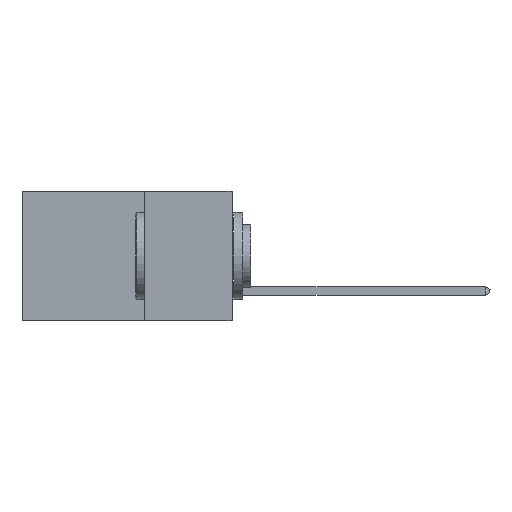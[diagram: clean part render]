
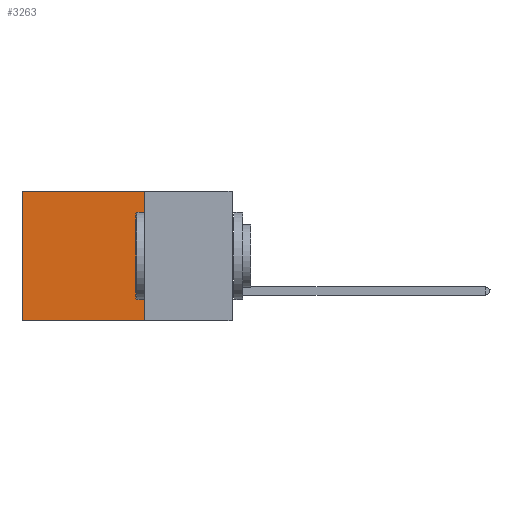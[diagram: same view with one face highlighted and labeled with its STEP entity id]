
A CAD part, left-side view. The second image highlights one B-rep face of the part: STEP entity #3263.
In plain terms, the highlighted planar face has unit normal (-1, 0, 0).
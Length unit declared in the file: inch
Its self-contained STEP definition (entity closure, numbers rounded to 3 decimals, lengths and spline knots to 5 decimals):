
#88 = VERTEX_POINT ( 'NONE', #1532 ) ;
#314 = EDGE_CURVE ( 'NONE', #6139, #6367, #6616, .T. ) ;
#353 = AXIS2_PLACEMENT_3D ( 'NONE', #1409, #7370, #13985 ) ;
#774 = EDGE_LOOP ( 'NONE', ( #6247, #1209, #3418, #14110 ) ) ;
#1006 = CARTESIAN_POINT ( 'NONE',  ( 0.2875, 0.25, 0. ) ) ;
#1209 = ORIENTED_EDGE ( 'NONE', *, *, #1333, .F. ) ;
#1333 = EDGE_CURVE ( 'NONE', #7862, #88, #13967, .T. ) ;
#1409 = CARTESIAN_POINT ( 'NONE',  ( 0.2875, 0.25, 0. ) ) ;
#1532 = CARTESIAN_POINT ( 'NONE',  ( 0.2875, 0.6, -0.37 ) ) ;
#1663 = DIRECTION ( 'NONE',  ( 0., 0., -1. ) ) ;
#1742 = VECTOR ( 'NONE', #6605, 39.37008 ) ;
#2166 = EDGE_CURVE ( 'NONE', #6139, #7862, #2516, .T. ) ;
#2516 = LINE ( 'NONE', #9166, #11994 ) ;
#2729 = CARTESIAN_POINT ( 'NONE',  ( 0.2875, 0.25, 0. ) ) ;
#2847 = CARTESIAN_POINT ( 'NONE',  ( 0.2875, 0.25, -0.37 ) ) ;
#3263 = ADVANCED_FACE ( 'NONE', ( #13203 ), #6681, .F. ) ;
#3418 = ORIENTED_EDGE ( 'NONE', *, *, #2166, .F. ) ;
#4540 = EDGE_CURVE ( 'NONE', #6367, #88, #7748, .T. ) ;
#4544 = VECTOR ( 'NONE', #9429, 39.37008 ) ;
#6139 = VERTEX_POINT ( 'NONE', #1006 ) ;
#6228 = DIRECTION ( 'NONE',  ( 0., 1., 0. ) ) ;
#6247 = ORIENTED_EDGE ( 'NONE', *, *, #4540, .T. ) ;
#6367 = VERTEX_POINT ( 'NONE', #10003 ) ;
#6605 = DIRECTION ( 'NONE',  ( 0., 0., -1. ) ) ;
#6616 = LINE ( 'NONE', #2729, #10501 ) ;
#6681 = PLANE ( 'NONE',  #353 ) ;
#7370 = DIRECTION ( 'NONE',  ( 1., 0., 0. ) ) ;
#7748 = LINE ( 'NONE', #9778, #1742 ) ;
#7862 = VERTEX_POINT ( 'NONE', #10607 ) ;
#9166 = CARTESIAN_POINT ( 'NONE',  ( 0.2875, 0.25, 0. ) ) ;
#9429 = DIRECTION ( 'NONE',  ( 0., 1., 0. ) ) ;
#9778 = CARTESIAN_POINT ( 'NONE',  ( 0.2875, 0.6, 0. ) ) ;
#10003 = CARTESIAN_POINT ( 'NONE',  ( 0.2875, 0.6, 0. ) ) ;
#10501 = VECTOR ( 'NONE', #6228, 39.37008 ) ;
#10607 = CARTESIAN_POINT ( 'NONE',  ( 0.2875, 0.25, -0.37 ) ) ;
#11994 = VECTOR ( 'NONE', #1663, 39.37008 ) ;
#13203 = FACE_OUTER_BOUND ( 'NONE', #774, .T. ) ;
#13967 = LINE ( 'NONE', #2847, #4544 ) ;
#13985 = DIRECTION ( 'NONE',  ( 0., 0., -1. ) ) ;
#14110 = ORIENTED_EDGE ( 'NONE', *, *, #314, .T. ) ;
